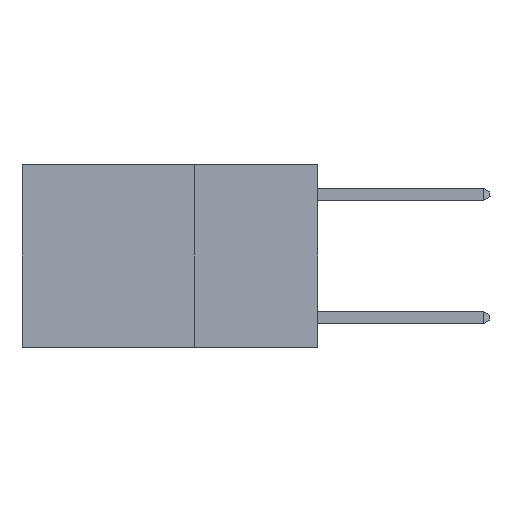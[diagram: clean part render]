
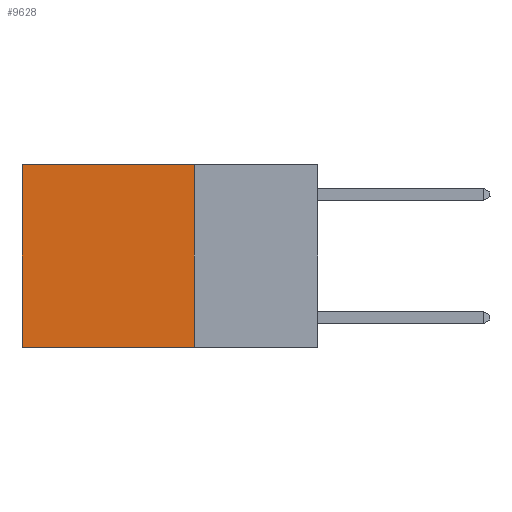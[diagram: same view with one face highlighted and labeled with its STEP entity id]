
A CAD part, left-side view. The second image highlights one B-rep face of the part: STEP entity #9628.
In plain terms, the highlighted planar face has unit normal (-1, 0, 0).
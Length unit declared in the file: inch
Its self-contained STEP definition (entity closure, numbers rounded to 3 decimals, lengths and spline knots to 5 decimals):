
#167 = VERTEX_POINT ( 'NONE', #2021 ) ;
#1512 = VERTEX_POINT ( 'NONE', #14803 ) ;
#2021 = CARTESIAN_POINT ( 'NONE',  ( 0.2625, 0.25, -0.37 ) ) ;
#2169 = EDGE_CURVE ( 'NONE', #1512, #167, #23181, .T. ) ;
#2242 = ORIENTED_EDGE ( 'NONE', *, *, #2169, .F. ) ;
#2434 = DIRECTION ( 'NONE',  ( 0., 1., 0. ) ) ;
#2649 = CARTESIAN_POINT ( 'NONE',  ( 0.2625, 0.6, 0. ) ) ;
#4893 = LINE ( 'NONE', #12747, #25176 ) ;
#5410 = VERTEX_POINT ( 'NONE', #19460 ) ;
#6378 = CARTESIAN_POINT ( 'NONE',  ( 0.2625, 0.25, 0. ) ) ;
#6553 = VECTOR ( 'NONE', #17316, 39.37008 ) ;
#7048 = DIRECTION ( 'NONE',  ( 0., 1., 0. ) ) ;
#7316 = EDGE_CURVE ( 'NONE', #167, #5410, #4893, .T. ) ;
#7595 = VERTEX_POINT ( 'NONE', #12447 ) ;
#9628 = ADVANCED_FACE ( 'NONE', ( #26825 ), #16816, .F. ) ;
#10264 = DIRECTION ( 'NONE',  ( 1., 0., 0. ) ) ;
#10570 = LINE ( 'NONE', #11148, #15132 ) ;
#10729 = CARTESIAN_POINT ( 'NONE',  ( 0.2625, 0.25, 0. ) ) ;
#11148 = CARTESIAN_POINT ( 'NONE',  ( 0.2625, 0.25, 0. ) ) ;
#12447 = CARTESIAN_POINT ( 'NONE',  ( 0.2625, 0.6, 0. ) ) ;
#12747 = CARTESIAN_POINT ( 'NONE',  ( 0.2625, 0.25, -0.37 ) ) ;
#14803 = CARTESIAN_POINT ( 'NONE',  ( 0.2625, 0.25, 0. ) ) ;
#14849 = ORIENTED_EDGE ( 'NONE', *, *, #7316, .F. ) ;
#15132 = VECTOR ( 'NONE', #2434, 39.37008 ) ;
#15184 = EDGE_CURVE ( 'NONE', #1512, #7595, #10570, .T. ) ;
#16816 = PLANE ( 'NONE',  #22199 ) ;
#17316 = DIRECTION ( 'NONE',  ( 0., 0., -1. ) ) ;
#17640 = VECTOR ( 'NONE', #25609, 39.37008 ) ;
#19460 = CARTESIAN_POINT ( 'NONE',  ( 0.2625, 0.6, -0.37 ) ) ;
#21275 = LINE ( 'NONE', #2649, #6553 ) ;
#21794 = EDGE_CURVE ( 'NONE', #7595, #5410, #21275, .T. ) ;
#22199 = AXIS2_PLACEMENT_3D ( 'NONE', #6378, #10264, #23115 ) ;
#22798 = ORIENTED_EDGE ( 'NONE', *, *, #15184, .T. ) ;
#23115 = DIRECTION ( 'NONE',  ( 0., 0., -1. ) ) ;
#23181 = LINE ( 'NONE', #10729, #17640 ) ;
#24309 = EDGE_LOOP ( 'NONE', ( #26239, #14849, #2242, #22798 ) ) ;
#25176 = VECTOR ( 'NONE', #7048, 39.37008 ) ;
#25609 = DIRECTION ( 'NONE',  ( 0., 0., -1. ) ) ;
#26239 = ORIENTED_EDGE ( 'NONE', *, *, #21794, .T. ) ;
#26825 = FACE_OUTER_BOUND ( 'NONE', #24309, .T. ) ;
